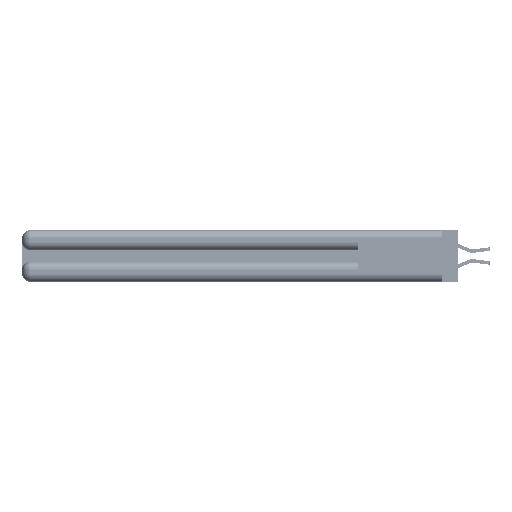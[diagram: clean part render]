
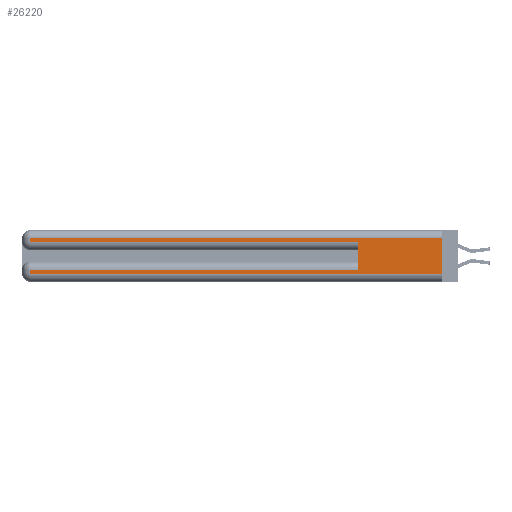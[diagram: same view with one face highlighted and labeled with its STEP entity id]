
A CAD part, left-side view. The second image highlights one B-rep face of the part: STEP entity #26220.
In plain terms, the highlighted planar face has unit normal (-1, 0, 0).
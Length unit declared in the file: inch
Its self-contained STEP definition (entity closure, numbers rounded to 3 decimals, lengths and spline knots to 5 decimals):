
#209 = DIRECTION ( 'NONE',  ( 0., 0., -1. ) ) ;
#1976 = ORIENTED_EDGE ( 'NONE', *, *, #7464, .T. ) ;
#2506 = CARTESIAN_POINT ( 'NONE',  ( 0., 0., 0.285 ) ) ;
#3119 = EDGE_CURVE ( 'NONE', #47627, #9326, #4164, .T. ) ;
#3991 = DIRECTION ( 'NONE',  ( 0., 1., 0. ) ) ;
#4164 = LINE ( 'NONE', #39420, #8096 ) ;
#4837 = FACE_OUTER_BOUND ( 'NONE', #10059, .T. ) ;
#5368 = PLANE ( 'NONE',  #24853 ) ;
#5703 = DIRECTION ( 'NONE',  ( 0., -1., 0. ) ) ;
#7464 = EDGE_CURVE ( 'NONE', #50610, #42863, #29510, .T. ) ;
#8096 = VECTOR ( 'NONE', #22030, 39.37008 ) ;
#9272 = CARTESIAN_POINT ( 'NONE',  ( 0., 2.94, 0.37 ) ) ;
#9326 = VERTEX_POINT ( 'NONE', #53822 ) ;
#10059 = EDGE_LOOP ( 'NONE', ( #14526, #50568, #27101, #38672, #50720, #38743, #11433, #1976 ) ) ;
#10186 = LINE ( 'NONE', #27051, #38963 ) ;
#10301 = CARTESIAN_POINT ( 'NONE',  ( 0., 0.6, 0.145 ) ) ;
#10444 = EDGE_CURVE ( 'NONE', #9326, #50610, #13499, .T. ) ;
#10696 = DIRECTION ( 'NONE',  ( 0., -1., 0. ) ) ;
#11255 = CARTESIAN_POINT ( 'NONE',  ( 0., 2.94, 0.06 ) ) ;
#11433 = ORIENTED_EDGE ( 'NONE', *, *, #10444, .T. ) ;
#12188 = VECTOR ( 'NONE', #3991, 39.37008 ) ;
#12828 = CARTESIAN_POINT ( 'NONE',  ( 0., 2.94, 0.37 ) ) ;
#13427 = DIRECTION ( 'NONE',  ( 0., 0., -1. ) ) ;
#13499 = LINE ( 'NONE', #9272, #39729 ) ;
#13612 = EDGE_CURVE ( 'NONE', #53277, #25417, #43041, .T. ) ;
#14526 = ORIENTED_EDGE ( 'NONE', *, *, #33749, .F. ) ;
#17047 = CARTESIAN_POINT ( 'NONE',  ( 0., 2.94, 0.31 ) ) ;
#18799 = VERTEX_POINT ( 'NONE', #49259 ) ;
#22030 = DIRECTION ( 'NONE',  ( 0., 1., 0. ) ) ;
#24485 = LINE ( 'NONE', #10301, #45433 ) ;
#24853 = AXIS2_PLACEMENT_3D ( 'NONE', #47293, #26059, #13427 ) ;
#24855 = CARTESIAN_POINT ( 'NONE',  ( 0., 0.6, 0.285 ) ) ;
#24970 = VECTOR ( 'NONE', #5703, 39.37008 ) ;
#25417 = VERTEX_POINT ( 'NONE', #17047 ) ;
#26059 = DIRECTION ( 'NONE',  ( 1., 0., 0. ) ) ;
#26220 = ADVANCED_FACE ( 'NONE', ( #4837 ), #5368, .F. ) ;
#26344 = EDGE_CURVE ( 'NONE', #47627, #53520, #24485, .T. ) ;
#27051 = CARTESIAN_POINT ( 'NONE',  ( 0., 0., 0.37 ) ) ;
#27101 = ORIENTED_EDGE ( 'NONE', *, *, #29405, .T. ) ;
#27489 = LINE ( 'NONE', #12828, #49113 ) ;
#28512 = CARTESIAN_POINT ( 'NONE',  ( 0., 0., 0.31 ) ) ;
#29405 = EDGE_CURVE ( 'NONE', #25417, #18799, #27489, .T. ) ;
#29510 = LINE ( 'NONE', #39000, #24970 ) ;
#30286 = DIRECTION ( 'NONE',  ( 0., 0., -1. ) ) ;
#30524 = DIRECTION ( 'NONE',  ( 0., 0., -1. ) ) ;
#31832 = CARTESIAN_POINT ( 'NONE',  ( 0., 0., 0.31 ) ) ;
#33749 = EDGE_CURVE ( 'NONE', #53277, #42863, #10186, .T. ) ;
#34536 = EDGE_CURVE ( 'NONE', #18799, #53520, #52726, .T. ) ;
#36719 = CARTESIAN_POINT ( 'NONE',  ( 0., 0., 0.06 ) ) ;
#38672 = ORIENTED_EDGE ( 'NONE', *, *, #34536, .T. ) ;
#38743 = ORIENTED_EDGE ( 'NONE', *, *, #3119, .T. ) ;
#38963 = VECTOR ( 'NONE', #30524, 39.37008 ) ;
#39000 = CARTESIAN_POINT ( 'NONE',  ( 0., 0., 0.06 ) ) ;
#39224 = DIRECTION ( 'NONE',  ( 0., 0., 1. ) ) ;
#39420 = CARTESIAN_POINT ( 'NONE',  ( 0., 0., 0.085 ) ) ;
#39729 = VECTOR ( 'NONE', #30286, 39.37008 ) ;
#42863 = VERTEX_POINT ( 'NONE', #36719 ) ;
#43041 = LINE ( 'NONE', #28512, #12188 ) ;
#44775 = VECTOR ( 'NONE', #10696, 39.37008 ) ;
#45433 = VECTOR ( 'NONE', #39224, 39.37008 ) ;
#47293 = CARTESIAN_POINT ( 'NONE',  ( 0., 0., 0.37 ) ) ;
#47627 = VERTEX_POINT ( 'NONE', #50349 ) ;
#49113 = VECTOR ( 'NONE', #209, 39.37008 ) ;
#49259 = CARTESIAN_POINT ( 'NONE',  ( 0., 2.94, 0.285 ) ) ;
#50349 = CARTESIAN_POINT ( 'NONE',  ( 0., 0.6, 0.085 ) ) ;
#50568 = ORIENTED_EDGE ( 'NONE', *, *, #13612, .T. ) ;
#50610 = VERTEX_POINT ( 'NONE', #11255 ) ;
#50720 = ORIENTED_EDGE ( 'NONE', *, *, #26344, .F. ) ;
#52726 = LINE ( 'NONE', #2506, #44775 ) ;
#53277 = VERTEX_POINT ( 'NONE', #31832 ) ;
#53520 = VERTEX_POINT ( 'NONE', #24855 ) ;
#53822 = CARTESIAN_POINT ( 'NONE',  ( 0., 2.94, 0.085 ) ) ;
